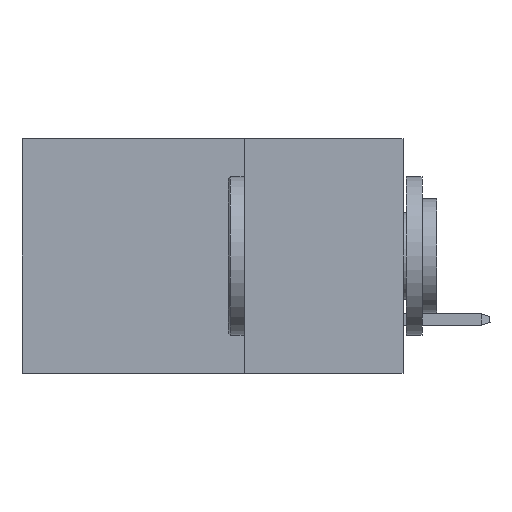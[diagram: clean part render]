
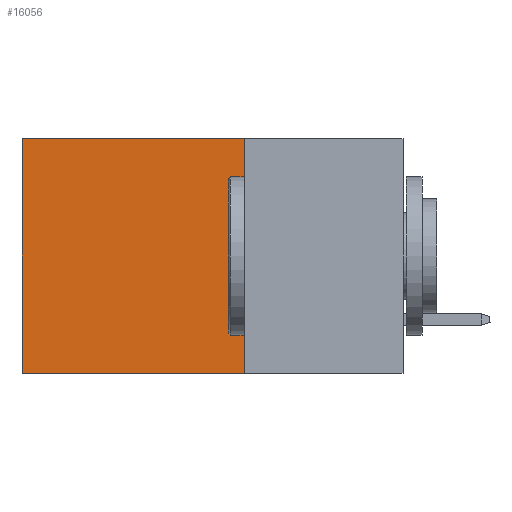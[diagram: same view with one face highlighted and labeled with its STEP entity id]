
A CAD part, left-side view. The second image highlights one B-rep face of the part: STEP entity #16056.
In plain terms, the highlighted planar face has unit normal (-1, 0, 0).
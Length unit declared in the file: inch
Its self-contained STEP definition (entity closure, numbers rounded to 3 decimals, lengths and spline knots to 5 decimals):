
#62 = DIRECTION ( 'NONE',  ( 0., 1., 0. ) ) ;
#1303 = ORIENTED_EDGE ( 'NONE', *, *, #19709, .F. ) ;
#2897 = DIRECTION ( 'NONE',  ( 0., 0., -1. ) ) ;
#3177 = EDGE_CURVE ( 'NONE', #17957, #42128, #10348, .T. ) ;
#4198 = AXIS2_PLACEMENT_3D ( 'NONE', #36669, #9048, #36017 ) ;
#6145 = ORIENTED_EDGE ( 'NONE', *, *, #22005, .F. ) ;
#6717 = VECTOR ( 'NONE', #21831, 39.37008 ) ;
#7695 = VECTOR ( 'NONE', #62, 39.37008 ) ;
#9048 = DIRECTION ( 'NONE',  ( 1., 0., 0. ) ) ;
#9929 = CARTESIAN_POINT ( 'NONE',  ( 0.2875, 0.25, -0.37 ) ) ;
#9990 = VERTEX_POINT ( 'NONE', #41716 ) ;
#10348 = LINE ( 'NONE', #20109, #7695 ) ;
#11969 = PLANE ( 'NONE',  #4198 ) ;
#13725 = LINE ( 'NONE', #9929, #27198 ) ;
#16056 = ADVANCED_FACE ( 'NONE', ( #28877 ), #11969, .F. ) ;
#17957 = VERTEX_POINT ( 'NONE', #33692 ) ;
#19128 = VERTEX_POINT ( 'NONE', #43557 ) ;
#19709 = EDGE_CURVE ( 'NONE', #19128, #9990, #13725, .T. ) ;
#20109 = CARTESIAN_POINT ( 'NONE',  ( 0.2875, 0.25, 0. ) ) ;
#20859 = VECTOR ( 'NONE', #2897, 39.37008 ) ;
#21628 = LINE ( 'NONE', #37925, #6717 ) ;
#21831 = DIRECTION ( 'NONE',  ( 0., 0., -1. ) ) ;
#22005 = EDGE_CURVE ( 'NONE', #17957, #19128, #27181, .T. ) ;
#27181 = LINE ( 'NONE', #40791, #20859 ) ;
#27198 = VECTOR ( 'NONE', #40244, 39.37008 ) ;
#28877 = FACE_OUTER_BOUND ( 'NONE', #43698, .T. ) ;
#33692 = CARTESIAN_POINT ( 'NONE',  ( 0.2875, 0.25, 0. ) ) ;
#36017 = DIRECTION ( 'NONE',  ( 0., 0., -1. ) ) ;
#36669 = CARTESIAN_POINT ( 'NONE',  ( 0.2875, 0.25, 0. ) ) ;
#37925 = CARTESIAN_POINT ( 'NONE',  ( 0.2875, 0.6, 0. ) ) ;
#39469 = CARTESIAN_POINT ( 'NONE',  ( 0.2875, 0.6, 0. ) ) ;
#39902 = EDGE_CURVE ( 'NONE', #42128, #9990, #21628, .T. ) ;
#40244 = DIRECTION ( 'NONE',  ( 0., 1., 0. ) ) ;
#40791 = CARTESIAN_POINT ( 'NONE',  ( 0.2875, 0.25, 0. ) ) ;
#41716 = CARTESIAN_POINT ( 'NONE',  ( 0.2875, 0.6, -0.37 ) ) ;
#41960 = ORIENTED_EDGE ( 'NONE', *, *, #39902, .T. ) ;
#42128 = VERTEX_POINT ( 'NONE', #39469 ) ;
#42646 = ORIENTED_EDGE ( 'NONE', *, *, #3177, .T. ) ;
#43557 = CARTESIAN_POINT ( 'NONE',  ( 0.2875, 0.25, -0.37 ) ) ;
#43698 = EDGE_LOOP ( 'NONE', ( #41960, #1303, #6145, #42646 ) ) ;
